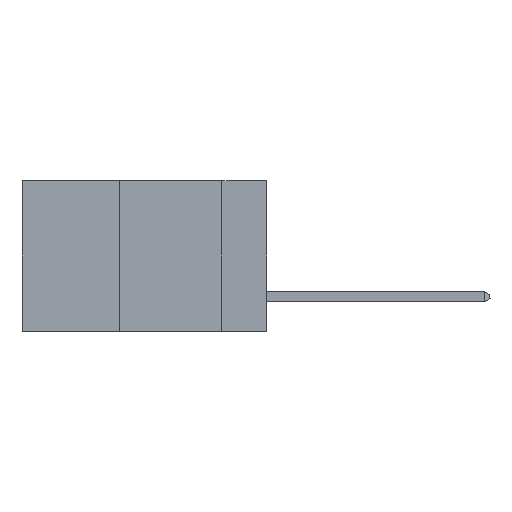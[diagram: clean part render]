
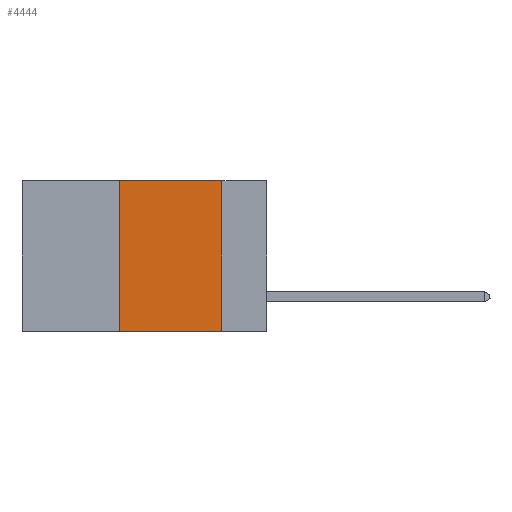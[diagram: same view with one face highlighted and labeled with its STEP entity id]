
A CAD part, left-side view. The second image highlights one B-rep face of the part: STEP entity #4444.
In plain terms, the highlighted planar face has unit normal (-1, 0, 0).
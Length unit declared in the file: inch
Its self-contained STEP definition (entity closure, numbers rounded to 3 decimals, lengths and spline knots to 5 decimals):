
#16 = ORIENTED_EDGE ( 'NONE', *, *, #1892, .F. ) ;
#142 = VECTOR ( 'NONE', #16705, 39.37008 ) ;
#1892 = EDGE_CURVE ( 'NONE', #11531, #16401, #20433, .T. ) ;
#2150 = ORIENTED_EDGE ( 'NONE', *, *, #10444, .F. ) ;
#3141 = CARTESIAN_POINT ( 'NONE',  ( 0., 0.11, 0. ) ) ;
#3425 = LINE ( 'NONE', #20763, #9315 ) ;
#3643 = CARTESIAN_POINT ( 'NONE',  ( 0., 0.11, -0.37 ) ) ;
#3848 = CARTESIAN_POINT ( 'NONE',  ( 0., 0.6, 0. ) ) ;
#4444 = ADVANCED_FACE ( 'NONE', ( #9317 ), #15874, .F. ) ;
#4472 = LINE ( 'NONE', #8687, #21813 ) ;
#5520 = DIRECTION ( 'NONE',  ( 0., -1., 0. ) ) ;
#5793 = DIRECTION ( 'NONE',  ( 1., 0., 0. ) ) ;
#5989 = ORIENTED_EDGE ( 'NONE', *, *, #11711, .T. ) ;
#6556 = VECTOR ( 'NONE', #12834, 39.37008 ) ;
#8326 = CARTESIAN_POINT ( 'NONE',  ( 0., 0.36, 0. ) ) ;
#8687 = CARTESIAN_POINT ( 'NONE',  ( 0., 0.36, 0. ) ) ;
#9315 = VECTOR ( 'NONE', #5520, 39.37008 ) ;
#9317 = FACE_OUTER_BOUND ( 'NONE', #16364, .T. ) ;
#10146 = AXIS2_PLACEMENT_3D ( 'NONE', #3848, #5793, #17578 ) ;
#10247 = DIRECTION ( 'NONE',  ( 0., 0., 1. ) ) ;
#10444 = EDGE_CURVE ( 'NONE', #19400, #11531, #3425, .T. ) ;
#11531 = VERTEX_POINT ( 'NONE', #11862 ) ;
#11711 = EDGE_CURVE ( 'NONE', #20248, #16401, #14982, .T. ) ;
#11862 = CARTESIAN_POINT ( 'NONE',  ( 0., 0.11, 0. ) ) ;
#12834 = DIRECTION ( 'NONE',  ( 0., -1., 0. ) ) ;
#14982 = LINE ( 'NONE', #17889, #6556 ) ;
#15874 = PLANE ( 'NONE',  #10146 ) ;
#16364 = EDGE_LOOP ( 'NONE', ( #16, #2150, #17669, #5989 ) ) ;
#16401 = VERTEX_POINT ( 'NONE', #3643 ) ;
#16705 = DIRECTION ( 'NONE',  ( 0., 0., -1. ) ) ;
#17578 = DIRECTION ( 'NONE',  ( 0., 0., -1. ) ) ;
#17669 = ORIENTED_EDGE ( 'NONE', *, *, #20417, .F. ) ;
#17889 = CARTESIAN_POINT ( 'NONE',  ( 0., 0.6, -0.37 ) ) ;
#19400 = VERTEX_POINT ( 'NONE', #8326 ) ;
#20248 = VERTEX_POINT ( 'NONE', #20352 ) ;
#20352 = CARTESIAN_POINT ( 'NONE',  ( 0., 0.36, -0.37 ) ) ;
#20417 = EDGE_CURVE ( 'NONE', #20248, #19400, #4472, .T. ) ;
#20433 = LINE ( 'NONE', #3141, #142 ) ;
#20763 = CARTESIAN_POINT ( 'NONE',  ( 0., 0.6, 0. ) ) ;
#21813 = VECTOR ( 'NONE', #10247, 39.37008 ) ;
